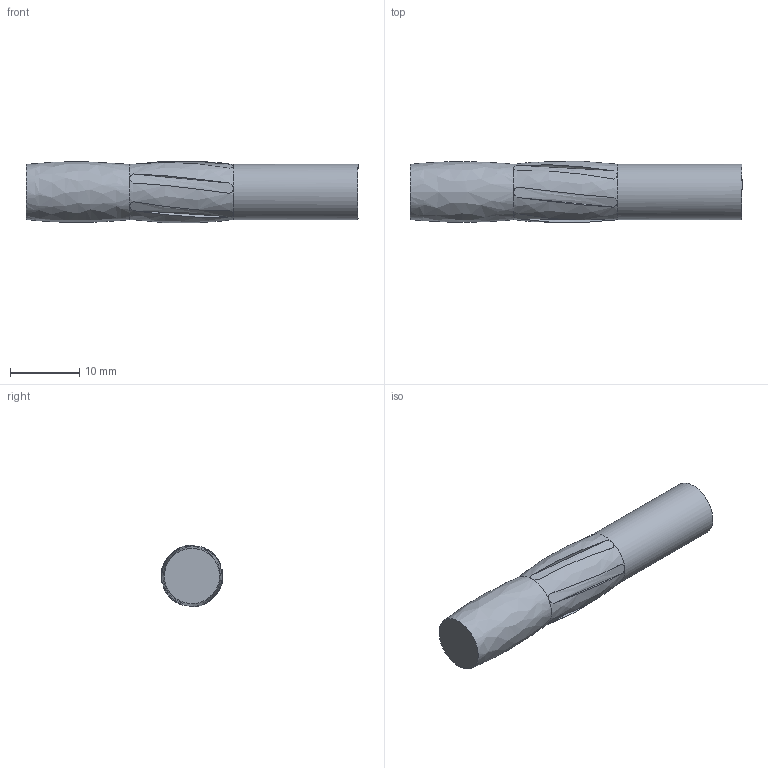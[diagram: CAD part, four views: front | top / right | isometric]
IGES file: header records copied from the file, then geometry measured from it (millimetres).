
Global section: file name: 9mm rifling button; native system: Autodesk Inventor 2019; preprocessor: unknown; author: user; date: 20200917.152551; units: millimetre
Bounding box: 48.03 x 8.88 x 8.92 mm (x, y, z)
Volume: 2608.8 mm3; surface area: 1415.5 mm2
Topology: 1 solids, 1 shells, 28 faces, 67 edges, 41 vertices
Faces by surface type: bspline 28
